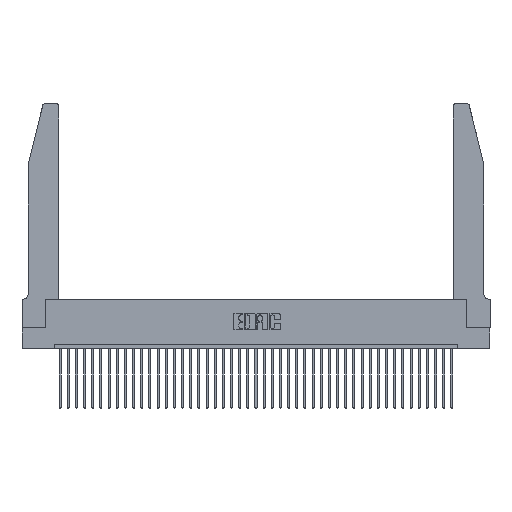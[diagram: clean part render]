
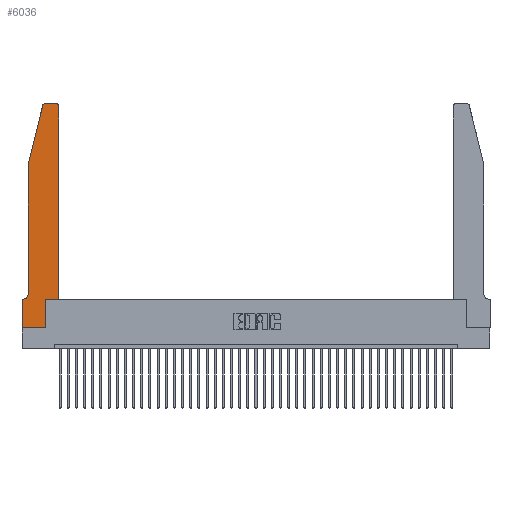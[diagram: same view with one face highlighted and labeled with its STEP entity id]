
A CAD part, top view. The second image highlights one B-rep face of the part: STEP entity #6036.
In plain terms, the highlighted planar face has unit normal (0, 0, 1).
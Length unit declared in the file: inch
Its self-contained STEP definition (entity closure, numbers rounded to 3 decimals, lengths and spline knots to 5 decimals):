
#296 = CARTESIAN_POINT ( 'NONE',  ( 0.4205, 2.72, 0.37 ) ) ;
#454 = VERTEX_POINT ( 'NONE', #35555 ) ;
#873 = EDGE_CURVE ( 'NONE', #35030, #454, #3014, .T. ) ;
#874 = DIRECTION ( 'NONE',  ( 0., -1., 0. ) ) ;
#934 = VECTOR ( 'NONE', #40603, 39.37008 ) ;
#1471 = ORIENTED_EDGE ( 'NONE', *, *, #7818, .T. ) ;
#2439 = EDGE_CURVE ( 'NONE', #14597, #39202, #32278, .T. ) ;
#3014 = LINE ( 'NONE', #9500, #5999 ) ;
#3202 = ORIENTED_EDGE ( 'NONE', *, *, #32314, .T. ) ;
#4141 = CARTESIAN_POINT ( 'NONE',  ( 0.0055, 0.35, 0.37 ) ) ;
#4899 = VERTEX_POINT ( 'NONE', #13317 ) ;
#5011 = LINE ( 'NONE', #35986, #33423 ) ;
#5613 = LINE ( 'NONE', #26644, #26695 ) ;
#5851 = CARTESIAN_POINT ( 'NONE',  ( 0.2865, 0.35, 0.37 ) ) ;
#5999 = VECTOR ( 'NONE', #31408, 39.37008 ) ;
#6036 = ADVANCED_FACE ( 'NONE', ( #25381 ), #31138, .T. ) ;
#6708 = AXIS2_PLACEMENT_3D ( 'NONE', #15765, #34288, #37350 ) ;
#6763 = ORIENTED_EDGE ( 'NONE', *, *, #20573, .T. ) ;
#6956 = CARTESIAN_POINT ( 'NONE',  ( 0.4505, 2.72, 0.37 ) ) ;
#7326 = DIRECTION ( 'NONE',  ( -1., 0., 0. ) ) ;
#7514 = ORIENTED_EDGE ( 'NONE', *, *, #9507, .T. ) ;
#7818 = EDGE_CURVE ( 'NONE', #454, #38043, #24263, .T. ) ;
#8476 = LINE ( 'NONE', #34604, #29529 ) ;
#8665 = CARTESIAN_POINT ( 'NONE',  ( 0.0755, 2., 0.37 ) ) ;
#9024 = VECTOR ( 'NONE', #21139, 39.37008 ) ;
#9283 = DIRECTION ( 'NONE',  ( 0., 0., 1. ) ) ;
#9471 = CIRCLE ( 'NONE', #24825, 0.03 ) ;
#9500 = CARTESIAN_POINT ( 'NONE',  ( 0.0755, 2., 0.37 ) ) ;
#9507 = EDGE_CURVE ( 'NONE', #37706, #28337, #5011, .T. ) ;
#10908 = DIRECTION ( 'NONE',  ( 1., 0., 0. ) ) ;
#13028 = CARTESIAN_POINT ( 'NONE',  ( 0.284, 2.72, 0.37 ) ) ;
#13317 = CARTESIAN_POINT ( 'NONE',  ( 0., 0., 0.37 ) ) ;
#13393 = DIRECTION ( 'NONE',  ( -1., 0., 0. ) ) ;
#13540 = ORIENTED_EDGE ( 'NONE', *, *, #2439, .T. ) ;
#13812 = CARTESIAN_POINT ( 'NONE',  ( 0.284, 2.75, 0.37 ) ) ;
#14041 = CARTESIAN_POINT ( 'NONE',  ( 0.4505, 0.35, 0.37 ) ) ;
#14285 = CARTESIAN_POINT ( 'NONE',  ( 0.25487, 2.72718, 0.37 ) ) ;
#14597 = VERTEX_POINT ( 'NONE', #24419 ) ;
#15257 = CARTESIAN_POINT ( 'NONE',  ( 0.2605, 2.75, 0.37 ) ) ;
#15765 = CARTESIAN_POINT ( 'NONE',  ( 0., 0.35, 0.37 ) ) ;
#16202 = DIRECTION ( 'NONE',  ( 0., 0., -1. ) ) ;
#16471 = CARTESIAN_POINT ( 'NONE',  ( 0.0055, 0.42, 0.37 ) ) ;
#17173 = DIRECTION ( 'NONE',  ( 0., 1., 0. ) ) ;
#17623 = EDGE_CURVE ( 'NONE', #4899, #14597, #5613, .T. ) ;
#17819 = VERTEX_POINT ( 'NONE', #4141 ) ;
#18103 = VERTEX_POINT ( 'NONE', #35382 ) ;
#18339 = VECTOR ( 'NONE', #10908, 39.37008 ) ;
#18631 = CARTESIAN_POINT ( 'NONE',  ( 0.0755, 0.35, 0.37 ) ) ;
#19053 = VECTOR ( 'NONE', #39191, 39.37008 ) ;
#20573 = EDGE_CURVE ( 'NONE', #18103, #27391, #34688, .T. ) ;
#20692 = CARTESIAN_POINT ( 'NONE',  ( 0., 0.35, 0.37 ) ) ;
#21139 = DIRECTION ( 'NONE',  ( 0., -1., 0. ) ) ;
#21784 = ORIENTED_EDGE ( 'NONE', *, *, #24262, .T. ) ;
#22563 = LINE ( 'NONE', #18631, #934 ) ;
#22946 = EDGE_CURVE ( 'NONE', #39202, #37706, #24730, .T. ) ;
#23343 = EDGE_CURVE ( 'NONE', #38043, #17819, #28168, .T. ) ;
#24262 = EDGE_CURVE ( 'NONE', #38470, #4899, #8476, .T. ) ;
#24263 = LINE ( 'NONE', #8665, #9024 ) ;
#24419 = CARTESIAN_POINT ( 'NONE',  ( 0.2865, 0., 0.37 ) ) ;
#24730 = LINE ( 'NONE', #14041, #18339 ) ;
#24825 = AXIS2_PLACEMENT_3D ( 'NONE', #296, #9283, #28191 ) ;
#25381 = FACE_OUTER_BOUND ( 'NONE', #38736, .T. ) ;
#25499 = ORIENTED_EDGE ( 'NONE', *, *, #22946, .T. ) ;
#26546 = CARTESIAN_POINT ( 'NONE',  ( 0.2865, 0.35, 0.37 ) ) ;
#26644 = CARTESIAN_POINT ( 'NONE',  ( 0., 0., 0.37 ) ) ;
#26695 = VECTOR ( 'NONE', #38995, 39.37008 ) ;
#27196 = ORIENTED_EDGE ( 'NONE', *, *, #873, .T. ) ;
#27391 = VERTEX_POINT ( 'NONE', #13812 ) ;
#27460 = ORIENTED_EDGE ( 'NONE', *, *, #40620, .T. ) ;
#28168 = CIRCLE ( 'NONE', #39403, 0.07 ) ;
#28191 = DIRECTION ( 'NONE',  ( 1., 0., 0. ) ) ;
#28337 = VERTEX_POINT ( 'NONE', #6956 ) ;
#29529 = VECTOR ( 'NONE', #874, 39.37008 ) ;
#31138 = PLANE ( 'NONE',  #6708 ) ;
#31181 = ORIENTED_EDGE ( 'NONE', *, *, #40700, .T. ) ;
#31408 = DIRECTION ( 'NONE',  ( -0.239, -0.971, 0. ) ) ;
#31632 = ORIENTED_EDGE ( 'NONE', *, *, #17623, .T. ) ;
#32278 = LINE ( 'NONE', #26546, #19053 ) ;
#32314 = EDGE_CURVE ( 'NONE', #28337, #18103, #9471, .T. ) ;
#33423 = VECTOR ( 'NONE', #17173, 39.37008 ) ;
#33914 = AXIS2_PLACEMENT_3D ( 'NONE', #13028, #38067, #35021 ) ;
#34288 = DIRECTION ( 'NONE',  ( 0., 0., 1. ) ) ;
#34604 = CARTESIAN_POINT ( 'NONE',  ( 0., 0., 0.37 ) ) ;
#34688 = LINE ( 'NONE', #15257, #40182 ) ;
#35021 = DIRECTION ( 'NONE',  ( 1., 0., 0. ) ) ;
#35030 = VERTEX_POINT ( 'NONE', #14285 ) ;
#35382 = CARTESIAN_POINT ( 'NONE',  ( 0.4205, 2.75, 0.37 ) ) ;
#35555 = CARTESIAN_POINT ( 'NONE',  ( 0.0755, 2., 0.37 ) ) ;
#35986 = CARTESIAN_POINT ( 'NONE',  ( 0.4505, 0.35, 0.37 ) ) ;
#36327 = ORIENTED_EDGE ( 'NONE', *, *, #23343, .T. ) ;
#37277 = CIRCLE ( 'NONE', #33914, 0.03 ) ;
#37350 = DIRECTION ( 'NONE',  ( 1., 0., 0. ) ) ;
#37599 = CARTESIAN_POINT ( 'NONE',  ( 0.0755, 0.42, 0.37 ) ) ;
#37706 = VERTEX_POINT ( 'NONE', #38878 ) ;
#38043 = VERTEX_POINT ( 'NONE', #37599 ) ;
#38067 = DIRECTION ( 'NONE',  ( 0., 0., 1. ) ) ;
#38470 = VERTEX_POINT ( 'NONE', #20692 ) ;
#38736 = EDGE_LOOP ( 'NONE', ( #6763, #31181, #27196, #1471, #36327, #27460, #21784, #31632, #13540, #25499, #7514, #3202 ) ) ;
#38878 = CARTESIAN_POINT ( 'NONE',  ( 0.4505, 0.35, 0.37 ) ) ;
#38995 = DIRECTION ( 'NONE',  ( 1., 0., 0. ) ) ;
#39191 = DIRECTION ( 'NONE',  ( 0., 1., 0. ) ) ;
#39202 = VERTEX_POINT ( 'NONE', #5851 ) ;
#39403 = AXIS2_PLACEMENT_3D ( 'NONE', #16471, #16202, #7326 ) ;
#40182 = VECTOR ( 'NONE', #13393, 39.37008 ) ;
#40603 = DIRECTION ( 'NONE',  ( -1., 0., 0. ) ) ;
#40620 = EDGE_CURVE ( 'NONE', #17819, #38470, #22563, .T. ) ;
#40700 = EDGE_CURVE ( 'NONE', #27391, #35030, #37277, .T. ) ;
